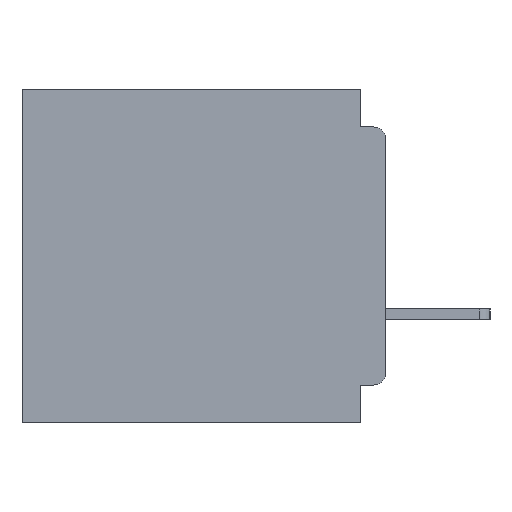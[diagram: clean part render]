
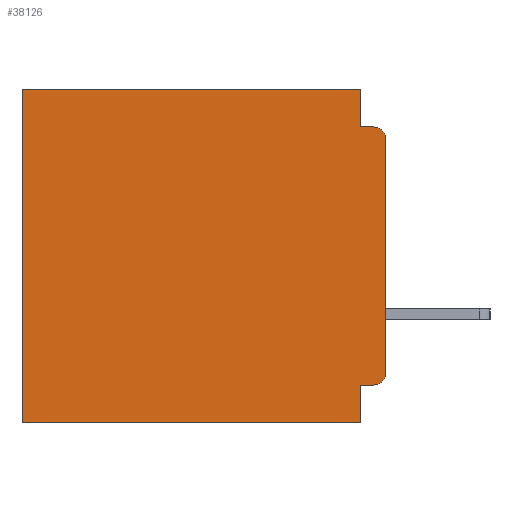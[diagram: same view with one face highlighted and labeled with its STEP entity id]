
A CAD part, left-side view. The second image highlights one B-rep face of the part: STEP entity #38126.
In plain terms, the highlighted planar face has unit normal (-1, 0, 0).
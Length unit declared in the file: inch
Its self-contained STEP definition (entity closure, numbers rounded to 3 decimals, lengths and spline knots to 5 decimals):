
#540 = ORIENTED_EDGE ( 'NONE', *, *, #17641, .T. ) ;
#616 = LINE ( 'NONE', #12491, #33996 ) ;
#1296 = CARTESIAN_POINT ( 'NONE',  ( 0.3, 0.031, 0. ) ) ;
#1577 = DIRECTION ( 'NONE',  ( 0., 0., -1. ) ) ;
#1712 = DIRECTION ( 'NONE',  ( 0., 0., -1. ) ) ;
#1800 = FACE_OUTER_BOUND ( 'NONE', #11819, .T. ) ;
#2073 = VECTOR ( 'NONE', #35070, 39.37008 ) ;
#2215 = CARTESIAN_POINT ( 'NONE',  ( 0.3, 0., -0.34 ) ) ;
#3336 = CARTESIAN_POINT ( 'NONE',  ( 0.3, 0.015, -0.355 ) ) ;
#3859 = EDGE_CURVE ( 'NONE', #12250, #16205, #6085, .T. ) ;
#4525 = AXIS2_PLACEMENT_3D ( 'NONE', #40435, #21084, #1712 ) ;
#4725 = CARTESIAN_POINT ( 'NONE',  ( 0.3, 0., -0.4 ) ) ;
#5028 = EDGE_CURVE ( 'NONE', #40470, #12250, #27303, .T. ) ;
#5457 = LINE ( 'NONE', #38018, #29308 ) ;
#5959 = ORIENTED_EDGE ( 'NONE', *, *, #35837, .F. ) ;
#6085 = LINE ( 'NONE', #26875, #39504 ) ;
#6477 = VECTOR ( 'NONE', #31384, 39.37008 ) ;
#7324 = VERTEX_POINT ( 'NONE', #13116 ) ;
#7989 = DIRECTION ( 'NONE',  ( 0., 0., -1. ) ) ;
#8369 = VERTEX_POINT ( 'NONE', #25363 ) ;
#8904 = VERTEX_POINT ( 'NONE', #1296 ) ;
#9563 = ORIENTED_EDGE ( 'NONE', *, *, #3859, .F. ) ;
#9838 = VERTEX_POINT ( 'NONE', #12670 ) ;
#10311 = DIRECTION ( 'NONE',  ( 0., 0., -1. ) ) ;
#11182 = VERTEX_POINT ( 'NONE', #36350 ) ;
#11819 = EDGE_LOOP ( 'NONE', ( #37977, #38913, #34360, #5959, #40376, #540, #25888, #9563, #12117, #38404 ) ) ;
#11974 = CARTESIAN_POINT ( 'NONE',  ( 0.3, 0., -0.4 ) ) ;
#12117 = ORIENTED_EDGE ( 'NONE', *, *, #5028, .F. ) ;
#12250 = VERTEX_POINT ( 'NONE', #33739 ) ;
#12491 = CARTESIAN_POINT ( 'NONE',  ( 0.3, 0., -0.4 ) ) ;
#12670 = CARTESIAN_POINT ( 'NONE',  ( 0.3, 0.015, -0.045 ) ) ;
#13116 = CARTESIAN_POINT ( 'NONE',  ( 0.3, 0.437, 0. ) ) ;
#14916 = CARTESIAN_POINT ( 'NONE',  ( 0.3, 0.031, -0.045 ) ) ;
#15390 = DIRECTION ( 'NONE',  ( 0., -1., 0. ) ) ;
#15709 = CARTESIAN_POINT ( 'NONE',  ( 0.3, 0.031, 0. ) ) ;
#15786 = VERTEX_POINT ( 'NONE', #2215 ) ;
#15967 = CARTESIAN_POINT ( 'NONE',  ( 0.3, 0., 0. ) ) ;
#16205 = VERTEX_POINT ( 'NONE', #33466 ) ;
#16278 = AXIS2_PLACEMENT_3D ( 'NONE', #40305, #20940, #1577 ) ;
#16465 = EDGE_CURVE ( 'NONE', #16205, #8369, #616, .T. ) ;
#17090 = CARTESIAN_POINT ( 'NONE',  ( 0.3, 0.437, -0.4 ) ) ;
#17641 = EDGE_CURVE ( 'NONE', #7324, #8369, #31387, .T. ) ;
#17840 = VERTEX_POINT ( 'NONE', #14916 ) ;
#18676 = VECTOR ( 'NONE', #41276, 39.37008 ) ;
#20940 = DIRECTION ( 'NONE',  ( -1., 0., 0. ) ) ;
#21064 = CIRCLE ( 'NONE', #4525, 0.015 ) ;
#21084 = DIRECTION ( 'NONE',  ( -1., 0., 0. ) ) ;
#23745 = LINE ( 'NONE', #11974, #6477 ) ;
#24023 = VECTOR ( 'NONE', #28858, 39.37008 ) ;
#24175 = PLANE ( 'NONE',  #27533 ) ;
#25068 = EDGE_CURVE ( 'NONE', #8904, #7324, #33611, .T. ) ;
#25363 = CARTESIAN_POINT ( 'NONE',  ( 0.3, 0.437, -0.4 ) ) ;
#25888 = ORIENTED_EDGE ( 'NONE', *, *, #16465, .F. ) ;
#26875 = CARTESIAN_POINT ( 'NONE',  ( 0.3, 0.031, -0.4 ) ) ;
#27303 = LINE ( 'NONE', #41657, #18676 ) ;
#27426 = DIRECTION ( 'NONE',  ( 1., 0., 0. ) ) ;
#27533 = AXIS2_PLACEMENT_3D ( 'NONE', #4725, #27426, #7989 ) ;
#28027 = EDGE_CURVE ( 'NONE', #11182, #9838, #35957, .T. ) ;
#28858 = DIRECTION ( 'NONE',  ( 0., 1., 0. ) ) ;
#28960 = LINE ( 'NONE', #15709, #2073 ) ;
#29308 = VECTOR ( 'NONE', #15390, 39.37008 ) ;
#31384 = DIRECTION ( 'NONE',  ( 0., 0., -1. ) ) ;
#31387 = LINE ( 'NONE', #17090, #40962 ) ;
#31826 = EDGE_CURVE ( 'NONE', #11182, #15786, #23745, .T. ) ;
#31869 = EDGE_CURVE ( 'NONE', #17840, #9838, #5457, .T. ) ;
#32945 = EDGE_CURVE ( 'NONE', #40470, #15786, #21064, .T. ) ;
#33466 = CARTESIAN_POINT ( 'NONE',  ( 0.3, 0.031, -0.4 ) ) ;
#33611 = LINE ( 'NONE', #15967, #24023 ) ;
#33739 = CARTESIAN_POINT ( 'NONE',  ( 0.3, 0.031, -0.355 ) ) ;
#33996 = VECTOR ( 'NONE', #35141, 39.37008 ) ;
#34360 = ORIENTED_EDGE ( 'NONE', *, *, #31869, .F. ) ;
#35070 = DIRECTION ( 'NONE',  ( 0., 0., -1. ) ) ;
#35141 = DIRECTION ( 'NONE',  ( 0., 1., 0. ) ) ;
#35837 = EDGE_CURVE ( 'NONE', #8904, #17840, #28960, .T. ) ;
#35957 = CIRCLE ( 'NONE', #16278, 0.015 ) ;
#36350 = CARTESIAN_POINT ( 'NONE',  ( 0.3, 0., -0.06 ) ) ;
#36456 = DIRECTION ( 'NONE',  ( 0., 0., -1. ) ) ;
#37977 = ORIENTED_EDGE ( 'NONE', *, *, #31826, .F. ) ;
#38018 = CARTESIAN_POINT ( 'NONE',  ( 0.3, 0., -0.045 ) ) ;
#38126 = ADVANCED_FACE ( 'NONE', ( #1800 ), #24175, .F. ) ;
#38404 = ORIENTED_EDGE ( 'NONE', *, *, #32945, .T. ) ;
#38913 = ORIENTED_EDGE ( 'NONE', *, *, #28027, .T. ) ;
#39504 = VECTOR ( 'NONE', #10311, 39.37008 ) ;
#40305 = CARTESIAN_POINT ( 'NONE',  ( 0.3, 0.015, -0.06 ) ) ;
#40376 = ORIENTED_EDGE ( 'NONE', *, *, #25068, .T. ) ;
#40435 = CARTESIAN_POINT ( 'NONE',  ( 0.3, 0.015, -0.34 ) ) ;
#40470 = VERTEX_POINT ( 'NONE', #3336 ) ;
#40962 = VECTOR ( 'NONE', #36456, 39.37008 ) ;
#41276 = DIRECTION ( 'NONE',  ( 0., 1., 0. ) ) ;
#41657 = CARTESIAN_POINT ( 'NONE',  ( 0.3, 0., -0.355 ) ) ;
